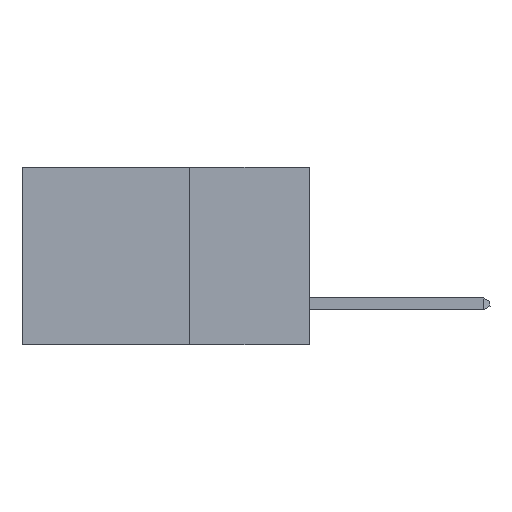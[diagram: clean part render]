
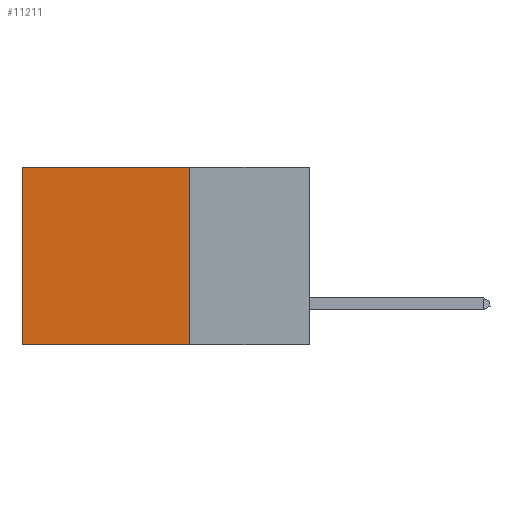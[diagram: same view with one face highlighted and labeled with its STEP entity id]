
A CAD part, left-side view. The second image highlights one B-rep face of the part: STEP entity #11211.
In plain terms, the highlighted planar face has unit normal (-1, 0, 0).
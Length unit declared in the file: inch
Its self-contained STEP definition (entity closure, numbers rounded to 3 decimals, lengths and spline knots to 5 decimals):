
#857 = VERTEX_POINT ( 'NONE', #20070 ) ;
#958 = VECTOR ( 'NONE', #19294, 39.37008 ) ;
#972 = ORIENTED_EDGE ( 'NONE', *, *, #4124, .F. ) ;
#1527 = CARTESIAN_POINT ( 'NONE',  ( 0.2875, 0.25, -0.37 ) ) ;
#4124 = EDGE_CURVE ( 'NONE', #5345, #16769, #25295, .T. ) ;
#4724 = VECTOR ( 'NONE', #13823, 39.37008 ) ;
#5016 = ORIENTED_EDGE ( 'NONE', *, *, #25377, .F. ) ;
#5313 = ORIENTED_EDGE ( 'NONE', *, *, #7845, .T. ) ;
#5345 = VERTEX_POINT ( 'NONE', #11379 ) ;
#6766 = LINE ( 'NONE', #7962, #18719 ) ;
#7736 = CARTESIAN_POINT ( 'NONE',  ( 0.2875, 0.6, -0.37 ) ) ;
#7845 = EDGE_CURVE ( 'NONE', #23083, #857, #11906, .T. ) ;
#7962 = CARTESIAN_POINT ( 'NONE',  ( 0.2875, 0.6, 0. ) ) ;
#8016 = DIRECTION ( 'NONE',  ( 0., 0., -1. ) ) ;
#8090 = DIRECTION ( 'NONE',  ( 1., 0., 0. ) ) ;
#11211 = ADVANCED_FACE ( 'NONE', ( #15790 ), #20067, .F. ) ;
#11379 = CARTESIAN_POINT ( 'NONE',  ( 0.2875, 0.25, -0.37 ) ) ;
#11906 = LINE ( 'NONE', #17331, #958 ) ;
#13823 = DIRECTION ( 'NONE',  ( 0., 1., 0. ) ) ;
#15790 = FACE_OUTER_BOUND ( 'NONE', #25810, .T. ) ;
#16071 = CARTESIAN_POINT ( 'NONE',  ( 0.2875, 0.25, 0. ) ) ;
#16143 = CARTESIAN_POINT ( 'NONE',  ( 0.2875, 0.25, 0. ) ) ;
#16769 = VERTEX_POINT ( 'NONE', #7736 ) ;
#17218 = LINE ( 'NONE', #16071, #21182 ) ;
#17331 = CARTESIAN_POINT ( 'NONE',  ( 0.2875, 0.25, 0. ) ) ;
#18057 = DIRECTION ( 'NONE',  ( 0., 0., -1. ) ) ;
#18719 = VECTOR ( 'NONE', #18057, 39.37008 ) ;
#18946 = ORIENTED_EDGE ( 'NONE', *, *, #19160, .T. ) ;
#19160 = EDGE_CURVE ( 'NONE', #857, #16769, #6766, .T. ) ;
#19294 = DIRECTION ( 'NONE',  ( 0., 1., 0. ) ) ;
#20067 = PLANE ( 'NONE',  #25987 ) ;
#20070 = CARTESIAN_POINT ( 'NONE',  ( 0.2875, 0.6, 0. ) ) ;
#21182 = VECTOR ( 'NONE', #8016, 39.37008 ) ;
#22025 = DIRECTION ( 'NONE',  ( 0., 0., -1. ) ) ;
#22150 = CARTESIAN_POINT ( 'NONE',  ( 0.2875, 0.25, 0. ) ) ;
#23083 = VERTEX_POINT ( 'NONE', #22150 ) ;
#25295 = LINE ( 'NONE', #1527, #4724 ) ;
#25377 = EDGE_CURVE ( 'NONE', #23083, #5345, #17218, .T. ) ;
#25810 = EDGE_LOOP ( 'NONE', ( #18946, #972, #5016, #5313 ) ) ;
#25987 = AXIS2_PLACEMENT_3D ( 'NONE', #16143, #8090, #22025 ) ;
